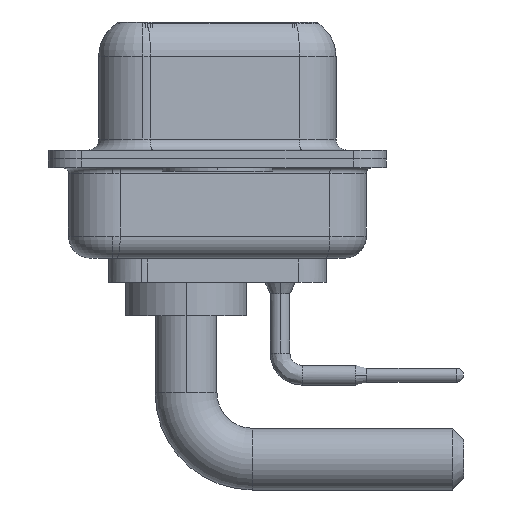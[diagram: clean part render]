
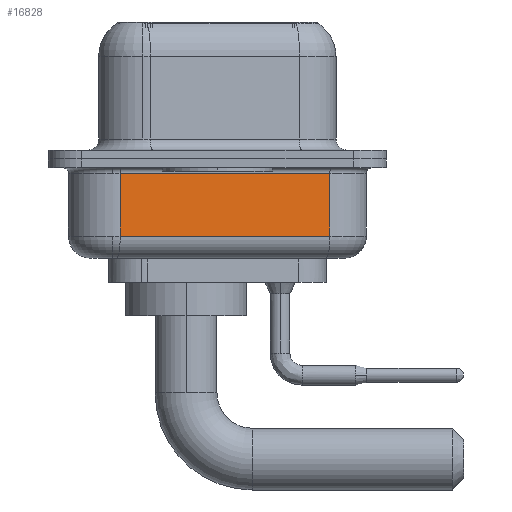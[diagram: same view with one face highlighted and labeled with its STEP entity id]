
A CAD part, left-side view. The second image highlights one B-rep face of the part: STEP entity #16828.
In plain terms, the highlighted planar face has unit normal (-0.985, -0.174, 0).
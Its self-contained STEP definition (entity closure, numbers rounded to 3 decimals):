
#864 = VERTEX_POINT ( 'NONE', #16015 ) ;
#2306 = CARTESIAN_POINT ( 'NONE',  ( 2.93, 4.403, -0.65 ) ) ;
#3438 = LINE ( 'NONE', #15451, #14907 ) ;
#3702 = AXIS2_PLACEMENT_3D ( 'NONE', #13015, #7187, #18988 ) ;
#4250 = FACE_OUTER_BOUND ( 'NONE', #4712, .T. ) ;
#4547 = LINE ( 'NONE', #7675, #9585 ) ;
#4712 = EDGE_LOOP ( 'NONE', ( #7136, #10748, #14478, #16956 ) ) ;
#4874 = CARTESIAN_POINT ( 'NONE',  ( 4.605, -5.097, -4.5 ) ) ;
#5039 = EDGE_CURVE ( 'NONE', #14543, #13596, #3438, .T. ) ;
#6987 = PLANE ( 'NONE',  #3702 ) ;
#7136 = ORIENTED_EDGE ( 'NONE', *, *, #5039, .F. ) ;
#7187 = DIRECTION ( 'NONE',  ( 0.985, 0.174, 0. ) ) ;
#7675 = CARTESIAN_POINT ( 'NONE',  ( 2.93, 4.403, -0.65 ) ) ;
#8014 = DIRECTION ( 'NONE',  ( 0., 0., 1. ) ) ;
#8929 = CARTESIAN_POINT ( 'NONE',  ( 2.93, 4.403, -3.5 ) ) ;
#9487 = LINE ( 'NONE', #4874, #17530 ) ;
#9585 = VECTOR ( 'NONE', #19177, 1000. ) ;
#10748 = ORIENTED_EDGE ( 'NONE', *, *, #15366, .T. ) ;
#11880 = LINE ( 'NONE', #8929, #17098 ) ;
#12975 = CARTESIAN_POINT ( 'NONE',  ( 2.93, 4.403, -3.5 ) ) ;
#13015 = CARTESIAN_POINT ( 'NONE',  ( 2.93, 4.403, -4.5 ) ) ;
#13596 = VERTEX_POINT ( 'NONE', #2306 ) ;
#14478 = ORIENTED_EDGE ( 'NONE', *, *, #19320, .T. ) ;
#14543 = VERTEX_POINT ( 'NONE', #12975 ) ;
#14907 = VECTOR ( 'NONE', #18469, 1000. ) ;
#15366 = EDGE_CURVE ( 'NONE', #14543, #864, #11880, .T. ) ;
#15432 = EDGE_CURVE ( 'NONE', #19343, #13596, #4547, .T. ) ;
#15451 = CARTESIAN_POINT ( 'NONE',  ( 2.93, 4.403, -4.5 ) ) ;
#16015 = CARTESIAN_POINT ( 'NONE',  ( 4.605, -5.097, -3.5 ) ) ;
#16828 = ADVANCED_FACE ( 'NONE', ( #4250 ), #6987, .F. ) ;
#16956 = ORIENTED_EDGE ( 'NONE', *, *, #15432, .T. ) ;
#17044 = CARTESIAN_POINT ( 'NONE',  ( 4.605, -5.097, -0.65 ) ) ;
#17098 = VECTOR ( 'NONE', #17777, 1000. ) ;
#17530 = VECTOR ( 'NONE', #8014, 1000. ) ;
#17777 = DIRECTION ( 'NONE',  ( 0.174, -0.985, 0. ) ) ;
#18469 = DIRECTION ( 'NONE',  ( 0., 0., 1. ) ) ;
#18988 = DIRECTION ( 'NONE',  ( -0.174, 0.985, 0. ) ) ;
#19177 = DIRECTION ( 'NONE',  ( -0.174, 0.985, 0. ) ) ;
#19320 = EDGE_CURVE ( 'NONE', #864, #19343, #9487, .T. ) ;
#19343 = VERTEX_POINT ( 'NONE', #17044 ) ;
